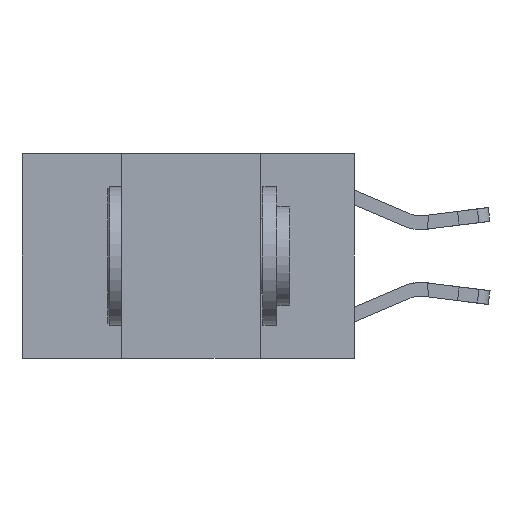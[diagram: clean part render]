
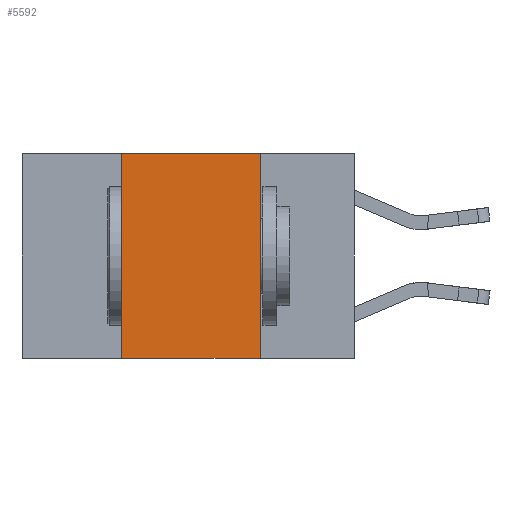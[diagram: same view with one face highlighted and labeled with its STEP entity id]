
A CAD part, left-side view. The second image highlights one B-rep face of the part: STEP entity #5592.
In plain terms, the highlighted planar face has unit normal (-1, 0, 0).
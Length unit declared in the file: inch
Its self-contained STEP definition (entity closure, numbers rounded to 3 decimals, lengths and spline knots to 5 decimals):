
#324 = DIRECTION ( 'NONE',  ( 0., 0., -1. ) ) ;
#483 = VECTOR ( 'NONE', #18191, 39.37008 ) ;
#1302 = ORIENTED_EDGE ( 'NONE', *, *, #26683, .T. ) ;
#2140 = VERTEX_POINT ( 'NONE', #26933 ) ;
#2947 = VERTEX_POINT ( 'NONE', #13674 ) ;
#2969 = ORIENTED_EDGE ( 'NONE', *, *, #14396, .F. ) ;
#4091 = EDGE_CURVE ( 'NONE', #2947, #27886, #16283, .T. ) ;
#4113 = FACE_OUTER_BOUND ( 'NONE', #17331, .T. ) ;
#4543 = DIRECTION ( 'NONE',  ( 0., 0., -1. ) ) ;
#5219 = ORIENTED_EDGE ( 'NONE', *, *, #25877, .F. ) ;
#5592 = ADVANCED_FACE ( 'NONE', ( #4113 ), #27873, .F. ) ;
#5883 = VECTOR ( 'NONE', #324, 39.37008 ) ;
#6810 = CARTESIAN_POINT ( 'NONE',  ( 0., 0.6, 0. ) ) ;
#8724 = VECTOR ( 'NONE', #27818, 39.37008 ) ;
#9342 = VERTEX_POINT ( 'NONE', #17394 ) ;
#9753 = CARTESIAN_POINT ( 'NONE',  ( 0., 0.6, -0.37 ) ) ;
#10959 = CARTESIAN_POINT ( 'NONE',  ( 0., 0.17, 0. ) ) ;
#11637 = CARTESIAN_POINT ( 'NONE',  ( 0., 0.6, 0. ) ) ;
#13403 = CARTESIAN_POINT ( 'NONE',  ( 0., 0.17, 0. ) ) ;
#13674 = CARTESIAN_POINT ( 'NONE',  ( 0., 0.42, 0. ) ) ;
#14156 = DIRECTION ( 'NONE',  ( 0., -1., 0. ) ) ;
#14396 = EDGE_CURVE ( 'NONE', #9342, #2947, #23562, .T. ) ;
#16283 = LINE ( 'NONE', #11637, #25501 ) ;
#17115 = DIRECTION ( 'NONE',  ( 1., 0., 0. ) ) ;
#17331 = EDGE_LOOP ( 'NONE', ( #5219, #26662, #2969, #1302 ) ) ;
#17394 = CARTESIAN_POINT ( 'NONE',  ( 0., 0.42, -0.37 ) ) ;
#18046 = LINE ( 'NONE', #9753, #483 ) ;
#18191 = DIRECTION ( 'NONE',  ( 0., -1., 0. ) ) ;
#23562 = LINE ( 'NONE', #25840, #8724 ) ;
#25501 = VECTOR ( 'NONE', #14156, 39.37008 ) ;
#25795 = LINE ( 'NONE', #10959, #5883 ) ;
#25840 = CARTESIAN_POINT ( 'NONE',  ( 0., 0.42, 0. ) ) ;
#25877 = EDGE_CURVE ( 'NONE', #27886, #2140, #25795, .T. ) ;
#26597 = AXIS2_PLACEMENT_3D ( 'NONE', #6810, #17115, #4543 ) ;
#26662 = ORIENTED_EDGE ( 'NONE', *, *, #4091, .F. ) ;
#26683 = EDGE_CURVE ( 'NONE', #9342, #2140, #18046, .T. ) ;
#26933 = CARTESIAN_POINT ( 'NONE',  ( 0., 0.17, -0.37 ) ) ;
#27818 = DIRECTION ( 'NONE',  ( 0., 0., 1. ) ) ;
#27873 = PLANE ( 'NONE',  #26597 ) ;
#27886 = VERTEX_POINT ( 'NONE', #13403 ) ;
